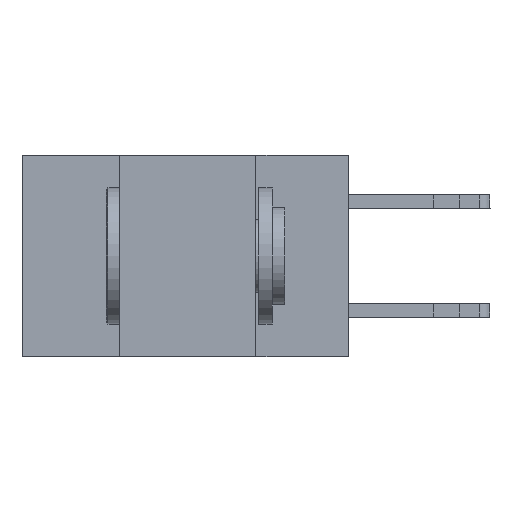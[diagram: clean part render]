
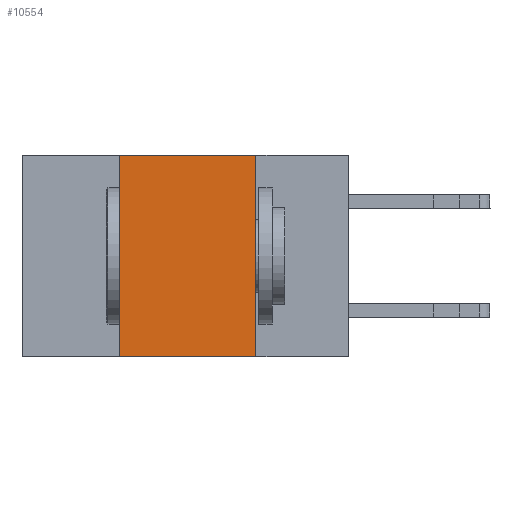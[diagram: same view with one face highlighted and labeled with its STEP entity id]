
A CAD part, left-side view. The second image highlights one B-rep face of the part: STEP entity #10554.
In plain terms, the highlighted planar face has unit normal (-1, 0, 0).
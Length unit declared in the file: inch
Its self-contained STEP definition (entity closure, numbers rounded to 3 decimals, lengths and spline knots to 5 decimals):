
#46 = DIRECTION ( 'NONE',  ( 1., 0., 0. ) ) ;
#237 = LINE ( 'NONE', #21248, #14478 ) ;
#444 = CARTESIAN_POINT ( 'NONE',  ( 0., 0.42, -0.37 ) ) ;
#1257 = DIRECTION ( 'NONE',  ( 0., 0., 1. ) ) ;
#1498 = AXIS2_PLACEMENT_3D ( 'NONE', #10777, #46, #12561 ) ;
#3227 = VERTEX_POINT ( 'NONE', #17913 ) ;
#4631 = EDGE_CURVE ( 'NONE', #7632, #19490, #21763, .T. ) ;
#5183 = EDGE_LOOP ( 'NONE', ( #20940, #19134, #20213, #20420 ) ) ;
#6031 = CARTESIAN_POINT ( 'NONE',  ( 0., 0.6, -0.37 ) ) ;
#6275 = VECTOR ( 'NONE', #20192, 39.37008 ) ;
#6826 = LINE ( 'NONE', #6031, #6275 ) ;
#7398 = VERTEX_POINT ( 'NONE', #444 ) ;
#7632 = VERTEX_POINT ( 'NONE', #21663 ) ;
#8992 = PLANE ( 'NONE',  #1498 ) ;
#10179 = CARTESIAN_POINT ( 'NONE',  ( 0., 0.42, -0.37 ) ) ;
#10554 = ADVANCED_FACE ( 'NONE', ( #20059 ), #8992, .F. ) ;
#10777 = CARTESIAN_POINT ( 'NONE',  ( 0., 0.6, 0. ) ) ;
#11010 = VECTOR ( 'NONE', #1257, 39.37008 ) ;
#11705 = VECTOR ( 'NONE', #14569, 39.37008 ) ;
#11774 = EDGE_CURVE ( 'NONE', #19490, #3227, #237, .T. ) ;
#12357 = DIRECTION ( 'NONE',  ( 0., 0., -1. ) ) ;
#12561 = DIRECTION ( 'NONE',  ( 0., 0., -1. ) ) ;
#14088 = CARTESIAN_POINT ( 'NONE',  ( 0., 0.17, 0. ) ) ;
#14478 = VECTOR ( 'NONE', #12357, 39.37008 ) ;
#14569 = DIRECTION ( 'NONE',  ( 0., -1., 0. ) ) ;
#14572 = CARTESIAN_POINT ( 'NONE',  ( 0., 0.6, 0. ) ) ;
#14589 = EDGE_CURVE ( 'NONE', #7398, #7632, #15745, .T. ) ;
#15745 = LINE ( 'NONE', #10179, #11010 ) ;
#17913 = CARTESIAN_POINT ( 'NONE',  ( 0., 0.17, -0.37 ) ) ;
#19134 = ORIENTED_EDGE ( 'NONE', *, *, #4631, .F. ) ;
#19490 = VERTEX_POINT ( 'NONE', #14088 ) ;
#19795 = EDGE_CURVE ( 'NONE', #7398, #3227, #6826, .T. ) ;
#20059 = FACE_OUTER_BOUND ( 'NONE', #5183, .T. ) ;
#20192 = DIRECTION ( 'NONE',  ( 0., -1., 0. ) ) ;
#20213 = ORIENTED_EDGE ( 'NONE', *, *, #14589, .F. ) ;
#20420 = ORIENTED_EDGE ( 'NONE', *, *, #19795, .T. ) ;
#20940 = ORIENTED_EDGE ( 'NONE', *, *, #11774, .F. ) ;
#21248 = CARTESIAN_POINT ( 'NONE',  ( 0., 0.17, -0.37 ) ) ;
#21663 = CARTESIAN_POINT ( 'NONE',  ( 0., 0.42, 0. ) ) ;
#21763 = LINE ( 'NONE', #14572, #11705 ) ;
